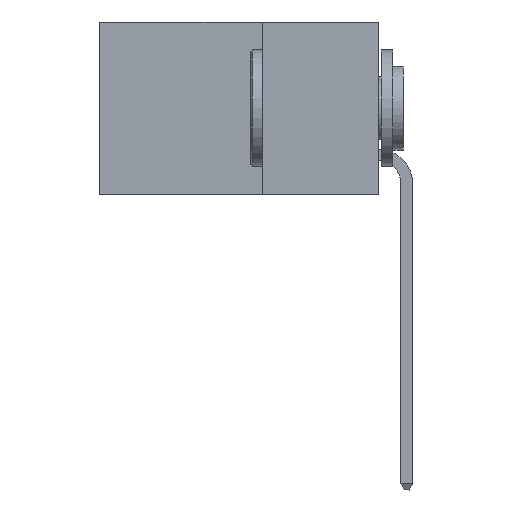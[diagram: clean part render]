
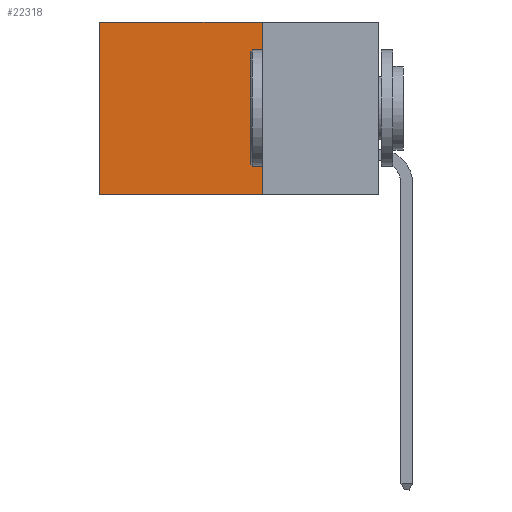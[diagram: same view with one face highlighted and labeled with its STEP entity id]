
A CAD part, left-side view. The second image highlights one B-rep face of the part: STEP entity #22318.
In plain terms, the highlighted planar face has unit normal (-1, 0, 0).
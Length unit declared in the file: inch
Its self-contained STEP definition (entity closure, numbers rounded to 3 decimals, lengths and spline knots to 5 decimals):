
#438 = ORIENTED_EDGE ( 'NONE', *, *, #2027, .F. ) ;
#832 = LINE ( 'NONE', #13771, #9285 ) ;
#846 = DIRECTION ( 'NONE',  ( 0., 0., -1. ) ) ;
#2027 = EDGE_CURVE ( 'NONE', #21641, #14569, #23262, .T. ) ;
#2208 = ORIENTED_EDGE ( 'NONE', *, *, #4702, .F. ) ;
#2983 = CARTESIAN_POINT ( 'NONE',  ( 0.298, 0.25, 0. ) ) ;
#3303 = CARTESIAN_POINT ( 'NONE',  ( 0.298, 0.25, -0.37 ) ) ;
#3670 = CARTESIAN_POINT ( 'NONE',  ( 0.298, 0.25, 0. ) ) ;
#4702 = EDGE_CURVE ( 'NONE', #14569, #8403, #20283, .T. ) ;
#4873 = CARTESIAN_POINT ( 'NONE',  ( 0.298, 0.25, 0. ) ) ;
#5441 = FACE_OUTER_BOUND ( 'NONE', #12148, .T. ) ;
#6928 = DIRECTION ( 'NONE',  ( 0., 1., 0. ) ) ;
#8105 = DIRECTION ( 'NONE',  ( 0., 0., -1. ) ) ;
#8403 = VERTEX_POINT ( 'NONE', #9357 ) ;
#8518 = CARTESIAN_POINT ( 'NONE',  ( 0.298, 0.6, 0. ) ) ;
#9284 = EDGE_CURVE ( 'NONE', #21641, #16969, #11784, .T. ) ;
#9285 = VECTOR ( 'NONE', #8105, 39.37008 ) ;
#9357 = CARTESIAN_POINT ( 'NONE',  ( 0.298, 0.6, -0.37 ) ) ;
#11784 = LINE ( 'NONE', #3670, #13761 ) ;
#12148 = EDGE_LOOP ( 'NONE', ( #18290, #2208, #438, #13202 ) ) ;
#12226 = PLANE ( 'NONE',  #15018 ) ;
#12303 = DIRECTION ( 'NONE',  ( 0., 0., -1. ) ) ;
#13202 = ORIENTED_EDGE ( 'NONE', *, *, #9284, .T. ) ;
#13652 = VECTOR ( 'NONE', #846, 39.37008 ) ;
#13761 = VECTOR ( 'NONE', #19884, 39.37008 ) ;
#13771 = CARTESIAN_POINT ( 'NONE',  ( 0.298, 0.6, 0. ) ) ;
#14109 = CARTESIAN_POINT ( 'NONE',  ( 0.298, 0.25, 0. ) ) ;
#14569 = VERTEX_POINT ( 'NONE', #15300 ) ;
#15018 = AXIS2_PLACEMENT_3D ( 'NONE', #14109, #17970, #12303 ) ;
#15189 = EDGE_CURVE ( 'NONE', #16969, #8403, #832, .T. ) ;
#15300 = CARTESIAN_POINT ( 'NONE',  ( 0.298, 0.25, -0.37 ) ) ;
#16896 = VECTOR ( 'NONE', #6928, 39.37008 ) ;
#16969 = VERTEX_POINT ( 'NONE', #8518 ) ;
#17970 = DIRECTION ( 'NONE',  ( 1., 0., 0. ) ) ;
#18290 = ORIENTED_EDGE ( 'NONE', *, *, #15189, .T. ) ;
#19884 = DIRECTION ( 'NONE',  ( 0., 1., 0. ) ) ;
#20283 = LINE ( 'NONE', #3303, #16896 ) ;
#21641 = VERTEX_POINT ( 'NONE', #4873 ) ;
#22318 = ADVANCED_FACE ( 'NONE', ( #5441 ), #12226, .F. ) ;
#23262 = LINE ( 'NONE', #2983, #13652 ) ;
